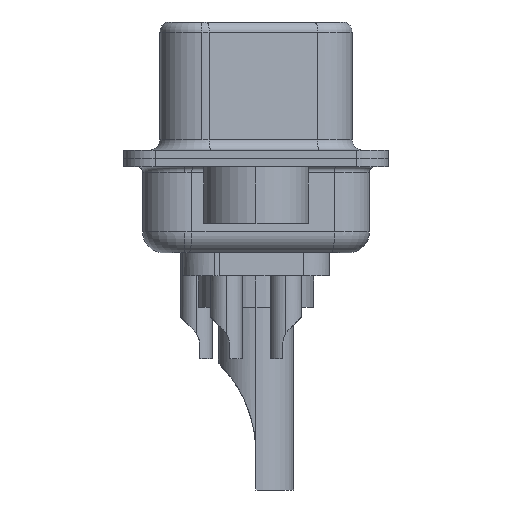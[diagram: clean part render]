
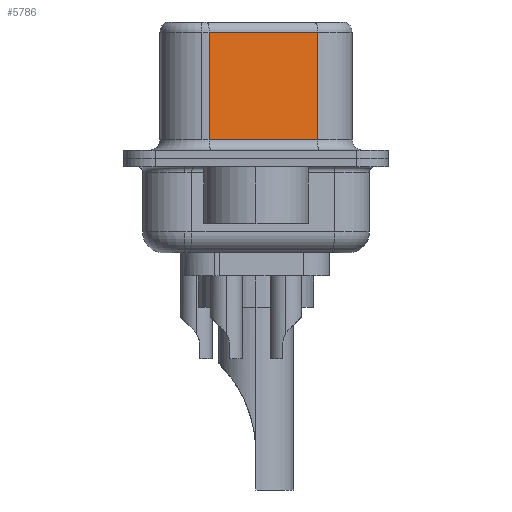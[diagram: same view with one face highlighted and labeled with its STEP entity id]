
A CAD part, left-side view. The second image highlights one B-rep face of the part: STEP entity #5786.
In plain terms, the highlighted planar face has unit normal (-0.985, -0.174, 0).
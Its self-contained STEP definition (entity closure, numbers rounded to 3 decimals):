
#413 = VERTEX_POINT ( 'NONE', #8885 ) ;
#1527 = CARTESIAN_POINT ( 'NONE',  ( 4.585, -2.927, 6.52 ) ) ;
#1528 = LINE ( 'NONE', #1527, #4924 ) ;
#2097 = CARTESIAN_POINT ( 'NONE',  ( 4.585, -2.927, 6.02 ) ) ;
#2425 = CARTESIAN_POINT ( 'NONE',  ( 3.675, 2.233, 0.9 ) ) ;
#3323 = CARTESIAN_POINT ( 'NONE',  ( 3.675, 2.233, 6.02 ) ) ;
#4123 = LINE ( 'NONE', #21000, #20445 ) ;
#4366 = VERTEX_POINT ( 'NONE', #2097 ) ;
#4682 = VECTOR ( 'NONE', #16965, 1000. ) ;
#4924 = VECTOR ( 'NONE', #17893, 1000. ) ;
#5024 = VERTEX_POINT ( 'NONE', #3323 ) ;
#5786 = ADVANCED_FACE ( 'NONE', ( #20739 ), #10026, .F. ) ;
#5933 = EDGE_CURVE ( 'NONE', #21433, #413, #23606, .T. ) ;
#6185 = CARTESIAN_POINT ( 'NONE',  ( 4.585, -2.927, 6.52 ) ) ;
#6269 = DIRECTION ( 'NONE',  ( -0.174, 0.985, 0. ) ) ;
#6283 = EDGE_CURVE ( 'NONE', #5024, #21433, #4123, .T. ) ;
#7648 = ORIENTED_EDGE ( 'NONE', *, *, #15772, .F. ) ;
#8885 = CARTESIAN_POINT ( 'NONE',  ( 4.585, -2.927, 0.9 ) ) ;
#10026 = PLANE ( 'NONE',  #17233 ) ;
#11464 = CARTESIAN_POINT ( 'NONE',  ( 4.585, -2.927, 0.9 ) ) ;
#14096 = EDGE_CURVE ( 'NONE', #4366, #5024, #18143, .T. ) ;
#15772 = EDGE_CURVE ( 'NONE', #4366, #413, #1528, .T. ) ;
#16085 = ORIENTED_EDGE ( 'NONE', *, *, #5933, .T. ) ;
#16965 = DIRECTION ( 'NONE',  ( -0.174, 0.985, 0. ) ) ;
#17233 = AXIS2_PLACEMENT_3D ( 'NONE', #6185, #20929, #6269 ) ;
#17519 = ORIENTED_EDGE ( 'NONE', *, *, #14096, .T. ) ;
#17615 = VECTOR ( 'NONE', #19977, 1000. ) ;
#17893 = DIRECTION ( 'NONE',  ( 0., 0., -1. ) ) ;
#18143 = LINE ( 'NONE', #22316, #4682 ) ;
#19882 = EDGE_LOOP ( 'NONE', ( #7648, #17519, #21120, #16085 ) ) ;
#19977 = DIRECTION ( 'NONE',  ( 0.174, -0.985, 0. ) ) ;
#20445 = VECTOR ( 'NONE', #22844, 1000. ) ;
#20739 = FACE_OUTER_BOUND ( 'NONE', #19882, .T. ) ;
#20929 = DIRECTION ( 'NONE',  ( 0.985, 0.174, 0. ) ) ;
#21000 = CARTESIAN_POINT ( 'NONE',  ( 3.675, 2.233, 6.52 ) ) ;
#21120 = ORIENTED_EDGE ( 'NONE', *, *, #6283, .T. ) ;
#21433 = VERTEX_POINT ( 'NONE', #2425 ) ;
#22316 = CARTESIAN_POINT ( 'NONE',  ( 4.585, -2.927, 6.02 ) ) ;
#22844 = DIRECTION ( 'NONE',  ( 0., 0., -1. ) ) ;
#23606 = LINE ( 'NONE', #11464, #17615 ) ;
